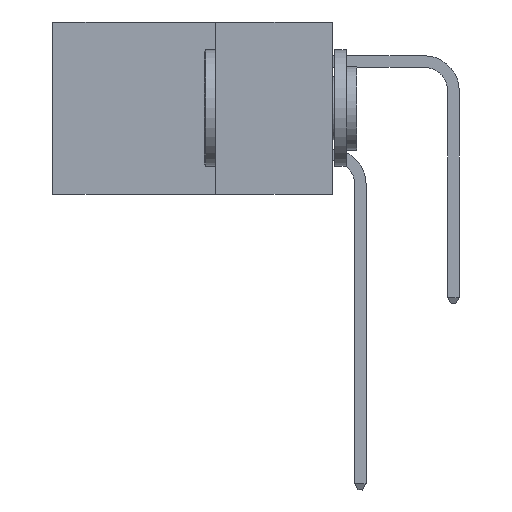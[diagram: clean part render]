
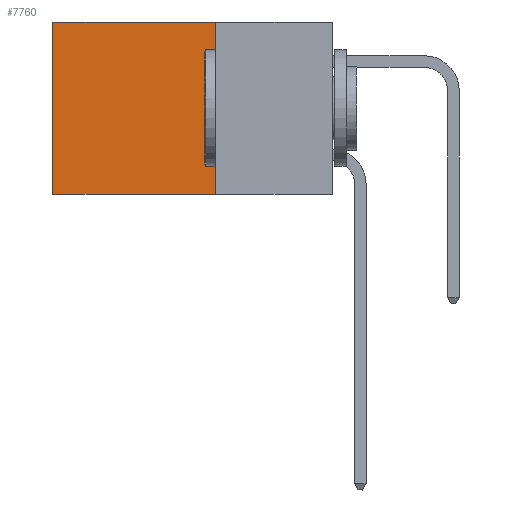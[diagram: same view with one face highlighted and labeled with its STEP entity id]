
A CAD part, left-side view. The second image highlights one B-rep face of the part: STEP entity #7760.
In plain terms, the highlighted planar face has unit normal (-1, 0, 0).
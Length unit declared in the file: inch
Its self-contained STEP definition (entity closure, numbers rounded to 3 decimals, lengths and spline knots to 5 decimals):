
#30 = LINE ( 'NONE', #10629, #9273 ) ;
#179 = FACE_OUTER_BOUND ( 'NONE', #9570, .T. ) ;
#285 = DIRECTION ( 'NONE',  ( 0., 1., 0. ) ) ;
#351 = AXIS2_PLACEMENT_3D ( 'NONE', #10080, #10911, #10834 ) ;
#1131 = VERTEX_POINT ( 'NONE', #8366 ) ;
#1898 = CARTESIAN_POINT ( 'NONE',  ( 0.298, 0.6, 0. ) ) ;
#1942 = ORIENTED_EDGE ( 'NONE', *, *, #9522, .T. ) ;
#2563 = ORIENTED_EDGE ( 'NONE', *, *, #6283, .F. ) ;
#2807 = VERTEX_POINT ( 'NONE', #9247 ) ;
#2970 = VECTOR ( 'NONE', #285, 39.37008 ) ;
#3623 = PLANE ( 'NONE',  #351 ) ;
#4453 = CARTESIAN_POINT ( 'NONE',  ( 0.298, 0.6, 0. ) ) ;
#4823 = LINE ( 'NONE', #4453, #5087 ) ;
#4840 = EDGE_CURVE ( 'NONE', #7583, #1131, #9889, .T. ) ;
#5037 = VERTEX_POINT ( 'NONE', #1898 ) ;
#5087 = VECTOR ( 'NONE', #9131, 39.37008 ) ;
#5537 = ORIENTED_EDGE ( 'NONE', *, *, #6677, .T. ) ;
#6283 = EDGE_CURVE ( 'NONE', #2807, #7583, #30, .T. ) ;
#6602 = VECTOR ( 'NONE', #6695, 39.37008 ) ;
#6677 = EDGE_CURVE ( 'NONE', #2807, #5037, #7249, .T. ) ;
#6695 = DIRECTION ( 'NONE',  ( 0., 1., 0. ) ) ;
#7249 = LINE ( 'NONE', #9387, #2970 ) ;
#7583 = VERTEX_POINT ( 'NONE', #10513 ) ;
#7760 = ADVANCED_FACE ( 'NONE', ( #179 ), #3623, .F. ) ;
#8366 = CARTESIAN_POINT ( 'NONE',  ( 0.298, 0.6, -0.37 ) ) ;
#9131 = DIRECTION ( 'NONE',  ( 0., 0., -1. ) ) ;
#9247 = CARTESIAN_POINT ( 'NONE',  ( 0.298, 0.25, 0. ) ) ;
#9273 = VECTOR ( 'NONE', #9816, 39.37008 ) ;
#9387 = CARTESIAN_POINT ( 'NONE',  ( 0.298, 0.25, 0. ) ) ;
#9522 = EDGE_CURVE ( 'NONE', #5037, #1131, #4823, .T. ) ;
#9570 = EDGE_LOOP ( 'NONE', ( #1942, #10106, #2563, #5537 ) ) ;
#9816 = DIRECTION ( 'NONE',  ( 0., 0., -1. ) ) ;
#9889 = LINE ( 'NONE', #10285, #6602 ) ;
#10080 = CARTESIAN_POINT ( 'NONE',  ( 0.298, 0.25, 0. ) ) ;
#10106 = ORIENTED_EDGE ( 'NONE', *, *, #4840, .F. ) ;
#10285 = CARTESIAN_POINT ( 'NONE',  ( 0.298, 0.25, -0.37 ) ) ;
#10513 = CARTESIAN_POINT ( 'NONE',  ( 0.298, 0.25, -0.37 ) ) ;
#10629 = CARTESIAN_POINT ( 'NONE',  ( 0.298, 0.25, 0. ) ) ;
#10834 = DIRECTION ( 'NONE',  ( 0., 0., -1. ) ) ;
#10911 = DIRECTION ( 'NONE',  ( 1., 0., 0. ) ) ;
